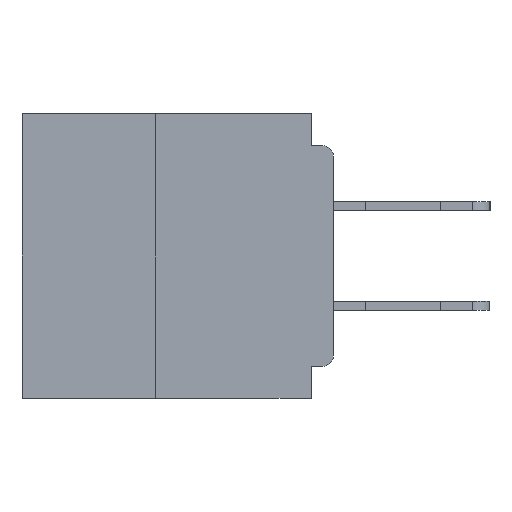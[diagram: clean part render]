
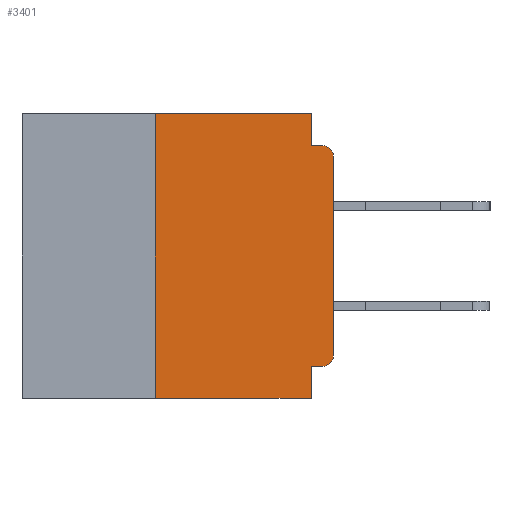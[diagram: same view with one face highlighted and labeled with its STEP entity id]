
A CAD part, left-side view. The second image highlights one B-rep face of the part: STEP entity #3401.
In plain terms, the highlighted planar face has unit normal (-1, 0, 0).
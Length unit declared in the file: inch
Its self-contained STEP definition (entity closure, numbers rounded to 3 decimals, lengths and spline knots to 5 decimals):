
#881 = CARTESIAN_POINT ( 'NONE',  ( 0., 0., -0.34 ) ) ;
#997 = LINE ( 'NONE', #1621, #43716 ) ;
#1202 = VECTOR ( 'NONE', #37482, 39.37008 ) ;
#1548 = ORIENTED_EDGE ( 'NONE', *, *, #36154, .F. ) ;
#1621 = CARTESIAN_POINT ( 'NONE',  ( 0., 0.031, -0.4 ) ) ;
#2649 = ORIENTED_EDGE ( 'NONE', *, *, #7951, .F. ) ;
#3401 = ADVANCED_FACE ( 'NONE', ( #25801 ), #22455, .F. ) ;
#3476 = DIRECTION ( 'NONE',  ( 0., 0., 1. ) ) ;
#4289 = ORIENTED_EDGE ( 'NONE', *, *, #21488, .T. ) ;
#4397 = CARTESIAN_POINT ( 'NONE',  ( 0., 0.25, -0.4 ) ) ;
#4696 = LINE ( 'NONE', #35946, #21998 ) ;
#4933 = VECTOR ( 'NONE', #3476, 39.37008 ) ;
#6616 = CARTESIAN_POINT ( 'NONE',  ( 0., 0.015, -0.34 ) ) ;
#7951 = EDGE_CURVE ( 'NONE', #10475, #17057, #8390, .T. ) ;
#8390 = LINE ( 'NONE', #41950, #16502 ) ;
#8512 = CARTESIAN_POINT ( 'NONE',  ( 0., 0.031, 0. ) ) ;
#9452 = VERTEX_POINT ( 'NONE', #22260 ) ;
#10107 = CARTESIAN_POINT ( 'NONE',  ( 0., 0.437, 0. ) ) ;
#10120 = DIRECTION ( 'NONE',  ( 0., 0., -1. ) ) ;
#10475 = VERTEX_POINT ( 'NONE', #31979 ) ;
#10512 = LINE ( 'NONE', #13366, #1202 ) ;
#11906 = LINE ( 'NONE', #4397, #29073 ) ;
#12488 = EDGE_CURVE ( 'NONE', #42634, #36410, #997, .T. ) ;
#13027 = ORIENTED_EDGE ( 'NONE', *, *, #33000, .F. ) ;
#13098 = CARTESIAN_POINT ( 'NONE',  ( 0., 0.25, -0.4 ) ) ;
#13366 = CARTESIAN_POINT ( 'NONE',  ( 0., 0.437, -0.4 ) ) ;
#13588 = ORIENTED_EDGE ( 'NONE', *, *, #12488, .F. ) ;
#14598 = ORIENTED_EDGE ( 'NONE', *, *, #22609, .T. ) ;
#15212 = DIRECTION ( 'NONE',  ( 0., 1., 0. ) ) ;
#16502 = VECTOR ( 'NONE', #24734, 39.37008 ) ;
#17056 = DIRECTION ( 'NONE',  ( -1., 0., 0. ) ) ;
#17057 = VERTEX_POINT ( 'NONE', #42899 ) ;
#18163 = VECTOR ( 'NONE', #32618, 39.37008 ) ;
#19424 = EDGE_CURVE ( 'NONE', #23179, #36410, #10512, .T. ) ;
#20312 = CARTESIAN_POINT ( 'NONE',  ( 0., 0.015, -0.355 ) ) ;
#20743 = AXIS2_PLACEMENT_3D ( 'NONE', #10107, #20839, #21295 ) ;
#20839 = DIRECTION ( 'NONE',  ( 1., 0., 0. ) ) ;
#21295 = DIRECTION ( 'NONE',  ( 0., 0., -1. ) ) ;
#21488 = EDGE_CURVE ( 'NONE', #27590, #27512, #23297, .T. ) ;
#21787 = CARTESIAN_POINT ( 'NONE',  ( 0., 0., -0.045 ) ) ;
#21998 = VECTOR ( 'NONE', #15212, 39.37008 ) ;
#22260 = CARTESIAN_POINT ( 'NONE',  ( 0., 0.015, -0.045 ) ) ;
#22455 = PLANE ( 'NONE',  #20743 ) ;
#22609 = EDGE_CURVE ( 'NONE', #27338, #27590, #36669, .T. ) ;
#22720 = CARTESIAN_POINT ( 'NONE',  ( 0., 0.031, -0.355 ) ) ;
#23179 = VERTEX_POINT ( 'NONE', #13098 ) ;
#23297 = LINE ( 'NONE', #27635, #4933 ) ;
#24734 = DIRECTION ( 'NONE',  ( 0., -1., 0. ) ) ;
#24896 = ORIENTED_EDGE ( 'NONE', *, *, #34916, .F. ) ;
#25109 = DIRECTION ( 'NONE',  ( 0., 0., 1. ) ) ;
#25801 = FACE_OUTER_BOUND ( 'NONE', #38687, .T. ) ;
#27192 = CIRCLE ( 'NONE', #31728, 0.015 ) ;
#27276 = LINE ( 'NONE', #8512, #18163 ) ;
#27338 = VERTEX_POINT ( 'NONE', #20312 ) ;
#27512 = VERTEX_POINT ( 'NONE', #41866 ) ;
#27590 = VERTEX_POINT ( 'NONE', #881 ) ;
#27635 = CARTESIAN_POINT ( 'NONE',  ( 0., 0., 0. ) ) ;
#29073 = VECTOR ( 'NONE', #25109, 39.37008 ) ;
#30750 = DIRECTION ( 'NONE',  ( -1., 0., 0. ) ) ;
#30835 = LINE ( 'NONE', #21787, #33016 ) ;
#31728 = AXIS2_PLACEMENT_3D ( 'NONE', #37673, #17056, #41146 ) ;
#31865 = EDGE_CURVE ( 'NONE', #38789, #9452, #30835, .T. ) ;
#31979 = CARTESIAN_POINT ( 'NONE',  ( 0., 0.25, 0. ) ) ;
#32618 = DIRECTION ( 'NONE',  ( 0., 0., -1. ) ) ;
#32793 = DIRECTION ( 'NONE',  ( 0., 0., -1. ) ) ;
#33000 = EDGE_CURVE ( 'NONE', #23179, #10475, #11906, .T. ) ;
#33016 = VECTOR ( 'NONE', #39128, 39.37008 ) ;
#33952 = AXIS2_PLACEMENT_3D ( 'NONE', #6616, #30750, #10120 ) ;
#34326 = CARTESIAN_POINT ( 'NONE',  ( 0., 0.031, -0.045 ) ) ;
#34916 = EDGE_CURVE ( 'NONE', #27338, #42634, #4696, .T. ) ;
#35946 = CARTESIAN_POINT ( 'NONE',  ( 0., 0., -0.355 ) ) ;
#36154 = EDGE_CURVE ( 'NONE', #17057, #38789, #27276, .T. ) ;
#36410 = VERTEX_POINT ( 'NONE', #37434 ) ;
#36669 = CIRCLE ( 'NONE', #33952, 0.015 ) ;
#37142 = EDGE_CURVE ( 'NONE', #27512, #9452, #27192, .T. ) ;
#37434 = CARTESIAN_POINT ( 'NONE',  ( 0., 0.031, -0.4 ) ) ;
#37482 = DIRECTION ( 'NONE',  ( 0., -1., 0. ) ) ;
#37673 = CARTESIAN_POINT ( 'NONE',  ( 0., 0.015, -0.06 ) ) ;
#37836 = ORIENTED_EDGE ( 'NONE', *, *, #19424, .T. ) ;
#38687 = EDGE_LOOP ( 'NONE', ( #4289, #41056, #43178, #1548, #2649, #13027, #37836, #13588, #24896, #14598 ) ) ;
#38789 = VERTEX_POINT ( 'NONE', #34326 ) ;
#39128 = DIRECTION ( 'NONE',  ( 0., -1., 0. ) ) ;
#41056 = ORIENTED_EDGE ( 'NONE', *, *, #37142, .T. ) ;
#41146 = DIRECTION ( 'NONE',  ( 0., 0., -1. ) ) ;
#41866 = CARTESIAN_POINT ( 'NONE',  ( 0., 0., -0.06 ) ) ;
#41950 = CARTESIAN_POINT ( 'NONE',  ( 0., 0.437, 0. ) ) ;
#42634 = VERTEX_POINT ( 'NONE', #22720 ) ;
#42899 = CARTESIAN_POINT ( 'NONE',  ( 0., 0.031, 0. ) ) ;
#43178 = ORIENTED_EDGE ( 'NONE', *, *, #31865, .F. ) ;
#43716 = VECTOR ( 'NONE', #32793, 39.37008 ) ;
